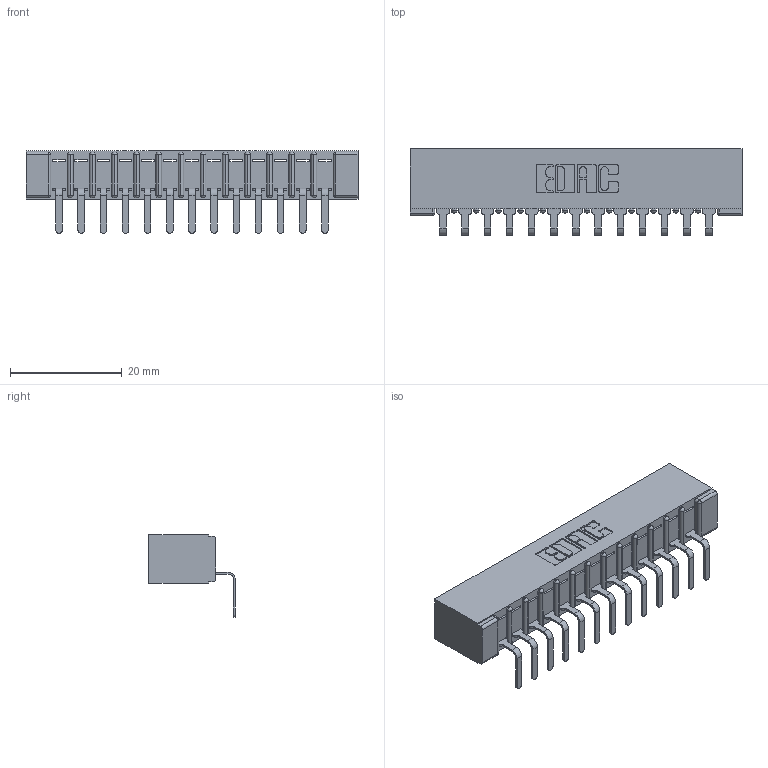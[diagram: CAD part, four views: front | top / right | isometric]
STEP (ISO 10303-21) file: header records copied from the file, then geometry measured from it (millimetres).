
FILE_DESCRIPTION (( 'STEP AP203' ), '1' );
FILE_NAME ('307-013-559-101.STEP', '2019-09-04T15:47:48', ( '' ), ( '' ), 'SwSTEP 2.0', 'SolidWorks 2016', '' );
FILE_SCHEMA (( 'CONFIG_CONTROL_DESIGN' ));
Length unit declared in the file: inch
Products named in the file (3): 307-013-559-101; 307 Part_No Mounting Lugs; 307-290-001_558 559 - 1 (Single)
Assembly tree (14 placements, depth 2):
  307-013-559-101
    307 Part_No Mounting Lugs
    307-290-001_558 559 - 1 (Single)  x13
Bounding box: 59.39 x 15.46 x 14.81 mm (x, y, z)
Volume: 3986.3 mm3; surface area: 6243.4 mm2
Topology: 14 solids, 14 shells, 904 faces, 2561 edges, 1650 vertices
Faces by surface type: plane 573, cylinder 303, sphere 28
Entity records: 14546 total; most frequent: CARTESIAN_POINT 2440, ORIENTED_EDGE 2426, DIRECTION 2389, EDGE_CURVE 1213, LINE 919, VECTOR 919, VERTEX_POINT 786, AXIS2_PLACEMENT_3D 735
